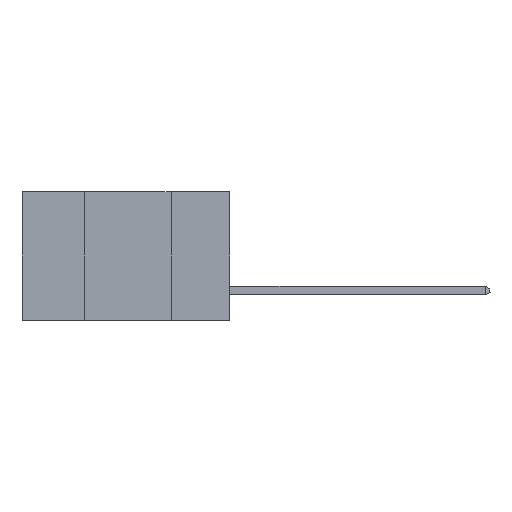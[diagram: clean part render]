
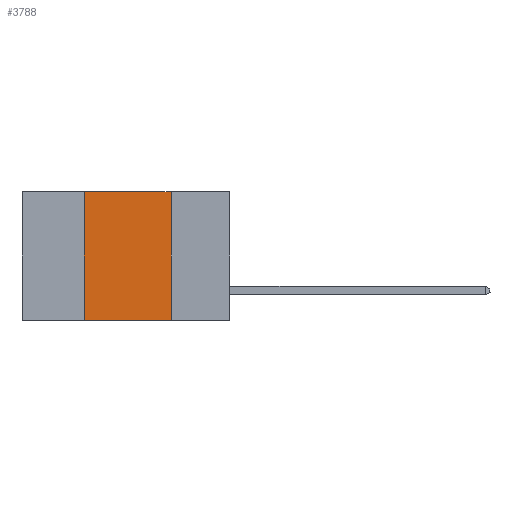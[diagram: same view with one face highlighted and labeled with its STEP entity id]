
A CAD part, left-side view. The second image highlights one B-rep face of the part: STEP entity #3788.
In plain terms, the highlighted planar face has unit normal (-1, 0, 0).
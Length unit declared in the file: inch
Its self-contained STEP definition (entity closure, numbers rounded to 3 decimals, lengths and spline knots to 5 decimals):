
#594 = DIRECTION ( 'NONE',  ( 0., -1., 0. ) ) ;
#2807 = VECTOR ( 'NONE', #24070, 39.37008 ) ;
#3196 = LINE ( 'NONE', #29794, #8187 ) ;
#3372 = VERTEX_POINT ( 'NONE', #29495 ) ;
#3410 = VERTEX_POINT ( 'NONE', #5483 ) ;
#3788 = ADVANCED_FACE ( 'NONE', ( #13957 ), #31397, .F. ) ;
#4367 = CARTESIAN_POINT ( 'NONE',  ( 0., 0.42, 0. ) ) ;
#4571 = EDGE_CURVE ( 'NONE', #11637, #3410, #23105, .T. ) ;
#4749 = ORIENTED_EDGE ( 'NONE', *, *, #9262, .F. ) ;
#4778 = DIRECTION ( 'NONE',  ( 0., -1., 0. ) ) ;
#5392 = VERTEX_POINT ( 'NONE', #17532 ) ;
#5483 = CARTESIAN_POINT ( 'NONE',  ( 0., 0.42, 0. ) ) ;
#7268 = DIRECTION ( 'NONE',  ( 1., 0., 0. ) ) ;
#7835 = DIRECTION ( 'NONE',  ( 0., 0., -1. ) ) ;
#7869 = CARTESIAN_POINT ( 'NONE',  ( 0., 0.42, -0.37 ) ) ;
#8187 = VECTOR ( 'NONE', #7835, 39.37008 ) ;
#8653 = ORIENTED_EDGE ( 'NONE', *, *, #4571, .F. ) ;
#9185 = CARTESIAN_POINT ( 'NONE',  ( 0., 0.6, 0. ) ) ;
#9262 = EDGE_CURVE ( 'NONE', #5392, #3372, #3196, .T. ) ;
#9450 = VECTOR ( 'NONE', #594, 39.37008 ) ;
#9837 = LINE ( 'NONE', #13172, #9450 ) ;
#10737 = ORIENTED_EDGE ( 'NONE', *, *, #13951, .T. ) ;
#11637 = VERTEX_POINT ( 'NONE', #7869 ) ;
#11697 = EDGE_LOOP ( 'NONE', ( #4749, #19476, #8653, #10737 ) ) ;
#13172 = CARTESIAN_POINT ( 'NONE',  ( 0., 0.6, -0.37 ) ) ;
#13951 = EDGE_CURVE ( 'NONE', #11637, #3372, #9837, .T. ) ;
#13957 = FACE_OUTER_BOUND ( 'NONE', #11697, .T. ) ;
#14488 = DIRECTION ( 'NONE',  ( 0., 0., -1. ) ) ;
#16934 = CARTESIAN_POINT ( 'NONE',  ( 0., 0.6, 0. ) ) ;
#17103 = AXIS2_PLACEMENT_3D ( 'NONE', #16934, #7268, #14488 ) ;
#17532 = CARTESIAN_POINT ( 'NONE',  ( 0., 0.17, 0. ) ) ;
#18701 = VECTOR ( 'NONE', #4778, 39.37008 ) ;
#19476 = ORIENTED_EDGE ( 'NONE', *, *, #24631, .F. ) ;
#21003 = LINE ( 'NONE', #9185, #18701 ) ;
#23105 = LINE ( 'NONE', #4367, #2807 ) ;
#24070 = DIRECTION ( 'NONE',  ( 0., 0., 1. ) ) ;
#24631 = EDGE_CURVE ( 'NONE', #3410, #5392, #21003, .T. ) ;
#29495 = CARTESIAN_POINT ( 'NONE',  ( 0., 0.17, -0.37 ) ) ;
#29794 = CARTESIAN_POINT ( 'NONE',  ( 0., 0.17, 0. ) ) ;
#31397 = PLANE ( 'NONE',  #17103 ) ;
